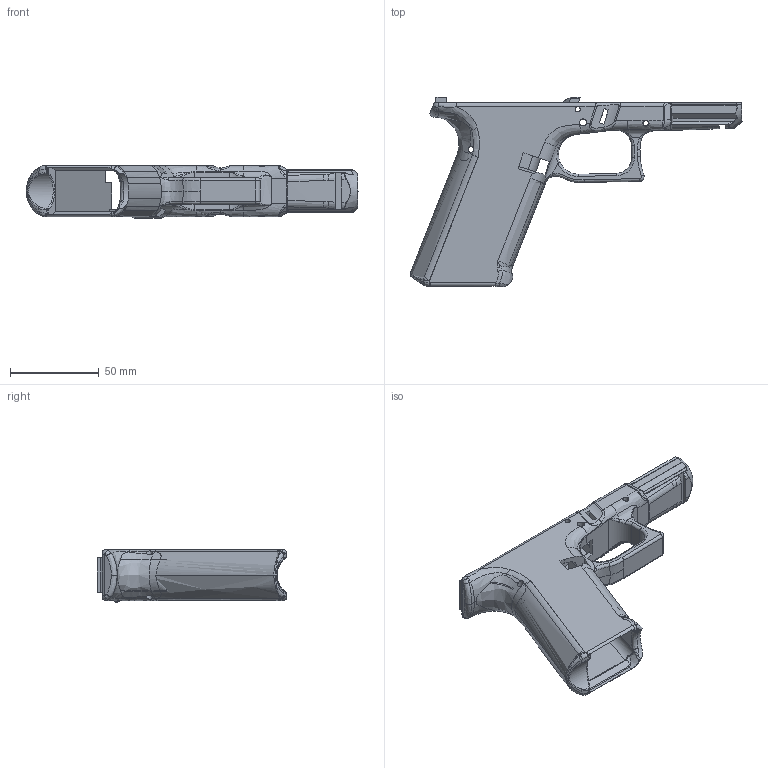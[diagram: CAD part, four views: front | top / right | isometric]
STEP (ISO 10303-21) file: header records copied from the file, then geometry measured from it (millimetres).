
FILE_DESCRIPTION(/* description */ (''),/* implementation_level */ '2;1');
FILE_NAME(/* name */ 'FMDA DD19x.2 v1.step',/* time_stamp */ '2022-12-21T20:41:37-07:00',/* author */ (''),/* organization */ (''),/* preprocessor_version */ 'ST-DEVELOPER v19.2',/* originating_system */ 'Autodesk Translation Framework v11.17.0.187',/* authorisation */ '');
FILE_SCHEMA (('AUTOMOTIVE_DESIGN { 1 0 10303 214 3 1 1 }'));
Products named in the file (1): FMDA DD19x.2
Bounding box: 186.96 x 106.5 x 29.84 mm (x, y, z)
Volume: 84355.7 mm3; surface area: 46181.1 mm2
Topology: 1 solids, 3 shells, 697 faces, 1959 edges, 1235 vertices
Faces by surface type: bspline 297, plane 199, cylinder 148, torus 31, cone 12, sphere 10
Full cylindrical faces by diameter (mm): 2 x1, 3 x4, 3.2 x2, 4 x2
Entity records: 53594 total; most frequent: CARTESIAN_POINT 37225, ORIENTED_EDGE 3890, DIRECTION 2761, EDGE_CURVE 1945, VERTEX_POINT 1236, AXIS2_PLACEMENT_3D 1016, LINE 729, VECTOR 729
